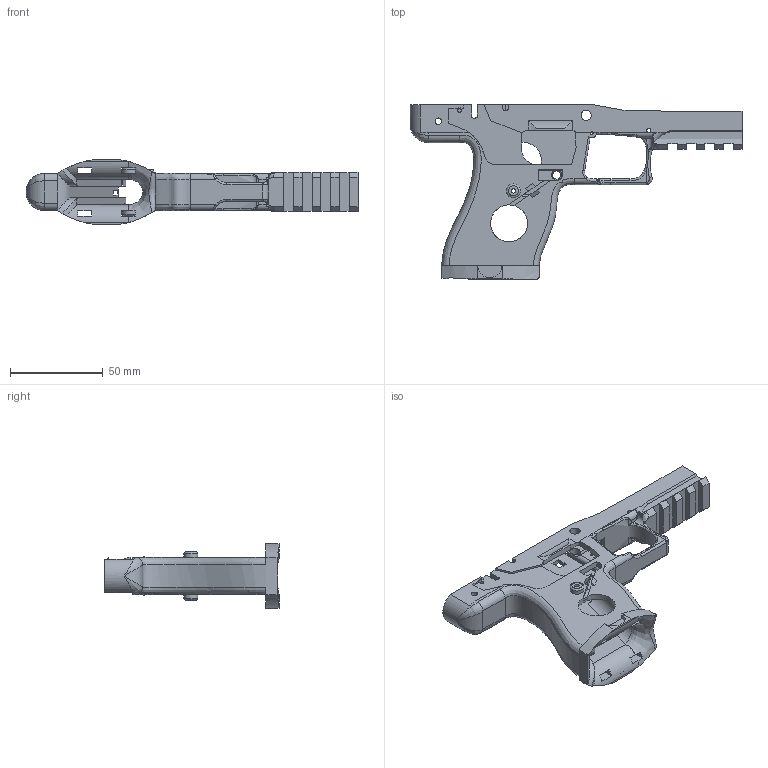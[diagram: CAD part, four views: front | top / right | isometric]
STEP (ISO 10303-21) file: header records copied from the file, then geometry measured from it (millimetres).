
FILE_DESCRIPTION(/* description */ (''),/* implementation_level */ '2;1');
FILE_NAME(/* name */ 'Freeman1337-lopointV2-1.0.step',/* time_stamp */ '2021-05-10T15:19:27-07:00',/* author */ (''),/* organization */ (''),/* preprocessor_version */ 'ST-DEVELOPER v18.1',/* originating_system */ 'Autodesk Translation Framework v10.6.0.1341',/* authorisation */ '');
FILE_SCHEMA (('AUTOMOTIVE_DESIGN { 1 0 10303 214 3 1 1 }'));
Length unit declared in the file: millimetre
Products named in the file (2): lopointV2-Frame; 0
Assembly tree (1 placements, depth 2):
  lopointV2-Frame
    0
Bounding box: 179 x 94.18 x 35 mm (x, y, z)
Volume: 74809.1 mm3; surface area: 38830 mm2
Topology: 1 solids, 1 shells, 2204 faces, 6321 edges, 4187 vertices
Faces by surface type: bspline 1582, plane 516, cylinder 95, torus 10, cone 1
Full cylindrical faces by diameter (mm): 1.5 x2, 2 x1, 2.2 x3, 2.4 x2, 3.5 x2, 3.7 x1, 4.4 x1, 5.5 x3, 6.5 x1, 6.75 x1, 7.5 x2, 20 x3
Entity records: 86808 total; most frequent: CARTESIAN_POINT 44022, ORIENTED_EDGE 12630, EDGE_CURVE 6315, DIRECTION 4553, VERTEX_POINT 4187, LINE 2805, VECTOR 2805, EDGE_LOOP 2332
